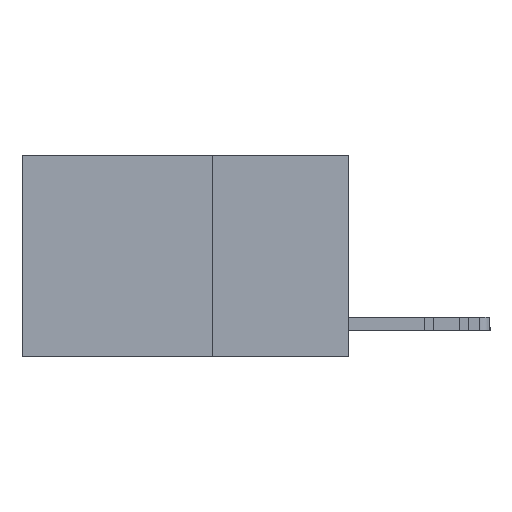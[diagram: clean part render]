
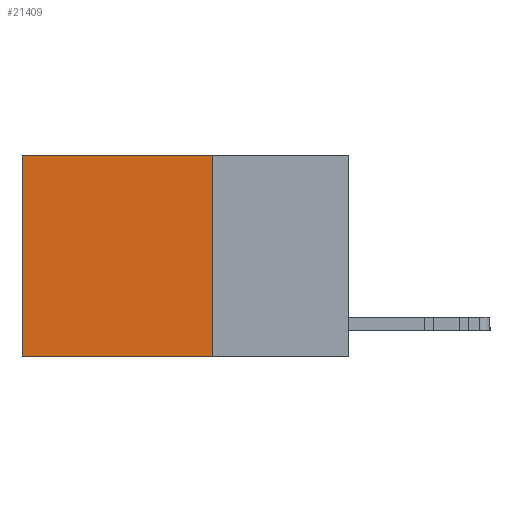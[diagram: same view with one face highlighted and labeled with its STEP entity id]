
A CAD part, left-side view. The second image highlights one B-rep face of the part: STEP entity #21409.
In plain terms, the highlighted planar face has unit normal (-1, 0, 0).
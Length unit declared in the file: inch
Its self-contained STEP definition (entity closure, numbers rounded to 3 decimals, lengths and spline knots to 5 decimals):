
#226 = DIRECTION ( 'NONE',  ( 0., 1., 0. ) ) ;
#307 = ORIENTED_EDGE ( 'NONE', *, *, #25314, .T. ) ;
#1792 = ORIENTED_EDGE ( 'NONE', *, *, #14406, .T. ) ;
#2641 = ORIENTED_EDGE ( 'NONE', *, *, #23748, .F. ) ;
#3897 = CARTESIAN_POINT ( 'NONE',  ( 0.2625, 0.25, -0.37 ) ) ;
#4005 = DIRECTION ( 'NONE',  ( 1., 0., 0. ) ) ;
#5992 = VECTOR ( 'NONE', #18503, 39.37008 ) ;
#7810 = LINE ( 'NONE', #23703, #5992 ) ;
#8454 = CARTESIAN_POINT ( 'NONE',  ( 0.2625, 0.25, 0. ) ) ;
#8749 = PLANE ( 'NONE',  #11766 ) ;
#9422 = VERTEX_POINT ( 'NONE', #26825 ) ;
#9558 = LINE ( 'NONE', #18622, #20876 ) ;
#11362 = EDGE_LOOP ( 'NONE', ( #1792, #16124, #2641, #307 ) ) ;
#11456 = LINE ( 'NONE', #16065, #26612 ) ;
#11548 = VERTEX_POINT ( 'NONE', #14627 ) ;
#11766 = AXIS2_PLACEMENT_3D ( 'NONE', #8454, #4005, #13035 ) ;
#12609 = CARTESIAN_POINT ( 'NONE',  ( 0.2625, 0.6, 0. ) ) ;
#13035 = DIRECTION ( 'NONE',  ( 0., 0., -1. ) ) ;
#14406 = EDGE_CURVE ( 'NONE', #19003, #9422, #7810, .T. ) ;
#14627 = CARTESIAN_POINT ( 'NONE',  ( 0.2625, 0.25, 0. ) ) ;
#15979 = LINE ( 'NONE', #20597, #16583 ) ;
#16065 = CARTESIAN_POINT ( 'NONE',  ( 0.2625, 0.25, 0. ) ) ;
#16124 = ORIENTED_EDGE ( 'NONE', *, *, #20217, .F. ) ;
#16583 = VECTOR ( 'NONE', #226, 39.37008 ) ;
#18503 = DIRECTION ( 'NONE',  ( 0., 0., -1. ) ) ;
#18622 = CARTESIAN_POINT ( 'NONE',  ( 0.2625, 0.25, 0. ) ) ;
#19003 = VERTEX_POINT ( 'NONE', #12609 ) ;
#20217 = EDGE_CURVE ( 'NONE', #24206, #9422, #15979, .T. ) ;
#20530 = DIRECTION ( 'NONE',  ( 0., 1., 0. ) ) ;
#20597 = CARTESIAN_POINT ( 'NONE',  ( 0.2625, 0.25, -0.37 ) ) ;
#20876 = VECTOR ( 'NONE', #27720, 39.37008 ) ;
#21409 = ADVANCED_FACE ( 'NONE', ( #29123 ), #8749, .F. ) ;
#23703 = CARTESIAN_POINT ( 'NONE',  ( 0.2625, 0.6, 0. ) ) ;
#23748 = EDGE_CURVE ( 'NONE', #11548, #24206, #9558, .T. ) ;
#24206 = VERTEX_POINT ( 'NONE', #3897 ) ;
#25314 = EDGE_CURVE ( 'NONE', #11548, #19003, #11456, .T. ) ;
#26612 = VECTOR ( 'NONE', #20530, 39.37008 ) ;
#26825 = CARTESIAN_POINT ( 'NONE',  ( 0.2625, 0.6, -0.37 ) ) ;
#27720 = DIRECTION ( 'NONE',  ( 0., 0., -1. ) ) ;
#29123 = FACE_OUTER_BOUND ( 'NONE', #11362, .T. ) ;
